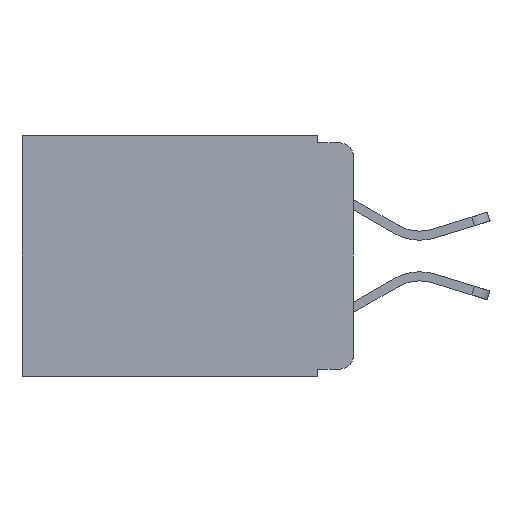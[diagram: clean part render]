
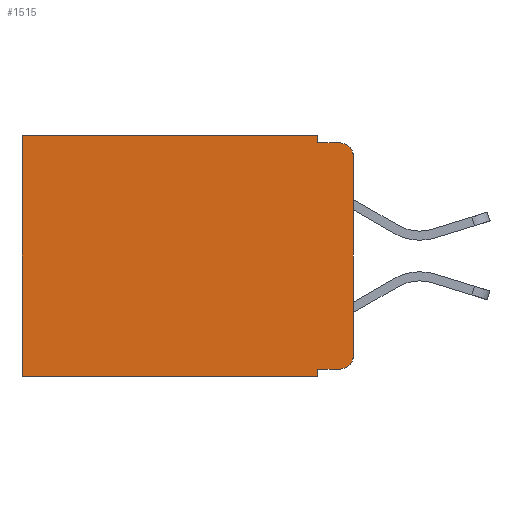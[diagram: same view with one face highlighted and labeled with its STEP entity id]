
A CAD part, left-side view. The second image highlights one B-rep face of the part: STEP entity #1515.
In plain terms, the highlighted planar face has unit normal (-1, 0, 0).
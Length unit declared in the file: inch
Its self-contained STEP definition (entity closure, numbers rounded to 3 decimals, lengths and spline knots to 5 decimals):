
#155 = VERTEX_POINT ( 'NONE', #9260 ) ;
#192 = VERTEX_POINT ( 'NONE', #7076 ) ;
#198 = DIRECTION ( 'NONE',  ( 1., 0., 0. ) ) ;
#301 = VECTOR ( 'NONE', #6604, 39.37008 ) ;
#324 = CARTESIAN_POINT ( 'NONE',  ( 0.298, 0., -0.313 ) ) ;
#326 = VERTEX_POINT ( 'NONE', #324 ) ;
#366 = ORIENTED_EDGE ( 'NONE', *, *, #368, .T. ) ;
#368 = EDGE_CURVE ( 'NONE', #2194, #5266, #1115, .T. ) ;
#650 = VECTOR ( 'NONE', #934, 39.37008 ) ;
#678 = CARTESIAN_POINT ( 'NONE',  ( 0.298, 0.02, -0.333 ) ) ;
#796 = VERTEX_POINT ( 'NONE', #10488 ) ;
#934 = DIRECTION ( 'NONE',  ( 0., 1., 0. ) ) ;
#1001 = DIRECTION ( 'NONE',  ( 0., 0., -1. ) ) ;
#1115 = CIRCLE ( 'NONE', #1779, 0.02 ) ;
#1192 = ORIENTED_EDGE ( 'NONE', *, *, #3396, .F. ) ;
#1207 = ORIENTED_EDGE ( 'NONE', *, *, #8757, .F. ) ;
#1311 = VERTEX_POINT ( 'NONE', #10526 ) ;
#1515 = ADVANCED_FACE ( 'NONE', ( #6422 ), #6947, .F. ) ;
#1528 = DIRECTION ( 'NONE',  ( 0., -1., 0. ) ) ;
#1566 = CARTESIAN_POINT ( 'NONE',  ( 0.298, 0.051, -0.01 ) ) ;
#1779 = AXIS2_PLACEMENT_3D ( 'NONE', #5170, #5738, #5725 ) ;
#1834 = ORIENTED_EDGE ( 'NONE', *, *, #7764, .T. ) ;
#1892 = LINE ( 'NONE', #10209, #8246 ) ;
#2194 = VERTEX_POINT ( 'NONE', #3260 ) ;
#2432 = CARTESIAN_POINT ( 'NONE',  ( 0.298, 0.473, 0. ) ) ;
#2502 = DIRECTION ( 'NONE',  ( -1., 0., 0. ) ) ;
#2789 = EDGE_CURVE ( 'NONE', #155, #796, #10693, .T. ) ;
#2820 = VECTOR ( 'NONE', #8921, 39.37008 ) ;
#3088 = AXIS2_PLACEMENT_3D ( 'NONE', #7680, #2502, #8460 ) ;
#3090 = EDGE_LOOP ( 'NONE', ( #3579, #366, #1207, #1192, #1834, #4958, #4820, #5309, #6899, #7160 ) ) ;
#3147 = VECTOR ( 'NONE', #1528, 39.37008 ) ;
#3260 = CARTESIAN_POINT ( 'NONE',  ( 0.298, 0., -0.03 ) ) ;
#3290 = VERTEX_POINT ( 'NONE', #5731 ) ;
#3396 = EDGE_CURVE ( 'NONE', #1311, #6406, #5147, .T. ) ;
#3579 = ORIENTED_EDGE ( 'NONE', *, *, #3991, .F. ) ;
#3657 = CIRCLE ( 'NONE', #3088, 0.02 ) ;
#3991 = EDGE_CURVE ( 'NONE', #2194, #326, #1892, .T. ) ;
#4078 = CARTESIAN_POINT ( 'NONE',  ( 0.298, 0.02, -0.01 ) ) ;
#4185 = VECTOR ( 'NONE', #8829, 39.37008 ) ;
#4287 = VECTOR ( 'NONE', #9888, 39.37008 ) ;
#4599 = CARTESIAN_POINT ( 'NONE',  ( 0.298, 0.051, 0. ) ) ;
#4820 = ORIENTED_EDGE ( 'NONE', *, *, #10430, .F. ) ;
#4958 = ORIENTED_EDGE ( 'NONE', *, *, #2789, .T. ) ;
#5140 = LINE ( 'NONE', #8175, #301 ) ;
#5147 = LINE ( 'NONE', #4599, #2820 ) ;
#5170 = CARTESIAN_POINT ( 'NONE',  ( 0.298, 0.02, -0.03 ) ) ;
#5266 = VERTEX_POINT ( 'NONE', #4078 ) ;
#5309 = ORIENTED_EDGE ( 'NONE', *, *, #7230, .F. ) ;
#5474 = CARTESIAN_POINT ( 'NONE',  ( 0.298, 0.051, 0. ) ) ;
#5725 = DIRECTION ( 'NONE',  ( 0., 0., -1. ) ) ;
#5731 = CARTESIAN_POINT ( 'NONE',  ( 0.298, 0.051, -0.333 ) ) ;
#5738 = DIRECTION ( 'NONE',  ( -1., 0., 0. ) ) ;
#6229 = DIRECTION ( 'NONE',  ( 0., 0., -1. ) ) ;
#6406 = VERTEX_POINT ( 'NONE', #10281 ) ;
#6422 = FACE_OUTER_BOUND ( 'NONE', #3090, .T. ) ;
#6604 = DIRECTION ( 'NONE',  ( 0., -1., 0. ) ) ;
#6811 = CARTESIAN_POINT ( 'NONE',  ( 0.298, 0., 0. ) ) ;
#6899 = ORIENTED_EDGE ( 'NONE', *, *, #10378, .T. ) ;
#6947 = PLANE ( 'NONE',  #7182 ) ;
#7076 = CARTESIAN_POINT ( 'NONE',  ( 0.298, 0.051, -0.343 ) ) ;
#7138 = LINE ( 'NONE', #9083, #4287 ) ;
#7160 = ORIENTED_EDGE ( 'NONE', *, *, #9896, .T. ) ;
#7182 = AXIS2_PLACEMENT_3D ( 'NONE', #6811, #198, #1001 ) ;
#7230 = EDGE_CURVE ( 'NONE', #3290, #192, #9583, .T. ) ;
#7473 = VECTOR ( 'NONE', #10301, 39.37008 ) ;
#7680 = CARTESIAN_POINT ( 'NONE',  ( 0.298, 0.02, -0.313 ) ) ;
#7764 = EDGE_CURVE ( 'NONE', #1311, #155, #9308, .T. ) ;
#8175 = CARTESIAN_POINT ( 'NONE',  ( 0.298, 0.051, -0.333 ) ) ;
#8246 = VECTOR ( 'NONE', #6229, 39.37008 ) ;
#8460 = DIRECTION ( 'NONE',  ( 0., 0., -1. ) ) ;
#8757 = EDGE_CURVE ( 'NONE', #6406, #5266, #9799, .T. ) ;
#8829 = DIRECTION ( 'NONE',  ( 0., 0., -1. ) ) ;
#8921 = DIRECTION ( 'NONE',  ( 0., 0., -1. ) ) ;
#9083 = CARTESIAN_POINT ( 'NONE',  ( 0.298, 0., -0.343 ) ) ;
#9260 = CARTESIAN_POINT ( 'NONE',  ( 0.298, 0.473, 0. ) ) ;
#9308 = LINE ( 'NONE', #9517, #650 ) ;
#9517 = CARTESIAN_POINT ( 'NONE',  ( 0.298, 0., 0. ) ) ;
#9583 = LINE ( 'NONE', #5474, #7473 ) ;
#9799 = LINE ( 'NONE', #1566, #3147 ) ;
#9888 = DIRECTION ( 'NONE',  ( 0., 1., 0. ) ) ;
#9896 = EDGE_CURVE ( 'NONE', #10911, #326, #3657, .T. ) ;
#10209 = CARTESIAN_POINT ( 'NONE',  ( 0.298, 0., 0. ) ) ;
#10281 = CARTESIAN_POINT ( 'NONE',  ( 0.298, 0.051, -0.01 ) ) ;
#10301 = DIRECTION ( 'NONE',  ( 0., 0., -1. ) ) ;
#10378 = EDGE_CURVE ( 'NONE', #3290, #10911, #5140, .T. ) ;
#10430 = EDGE_CURVE ( 'NONE', #192, #796, #7138, .T. ) ;
#10488 = CARTESIAN_POINT ( 'NONE',  ( 0.298, 0.473, -0.343 ) ) ;
#10526 = CARTESIAN_POINT ( 'NONE',  ( 0.298, 0.051, 0. ) ) ;
#10693 = LINE ( 'NONE', #2432, #4185 ) ;
#10911 = VERTEX_POINT ( 'NONE', #678 ) ;
